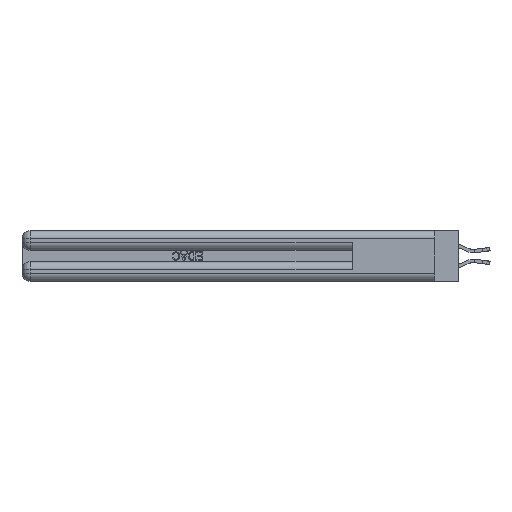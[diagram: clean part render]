
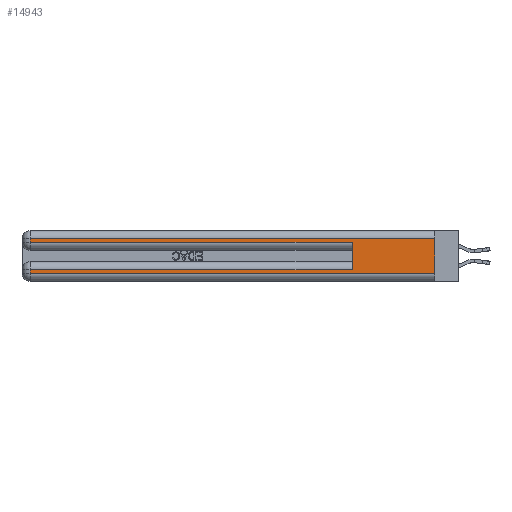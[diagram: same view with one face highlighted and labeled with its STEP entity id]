
A CAD part, left-side view. The second image highlights one B-rep face of the part: STEP entity #14943.
In plain terms, the highlighted planar face has unit normal (-1, 0, 0).
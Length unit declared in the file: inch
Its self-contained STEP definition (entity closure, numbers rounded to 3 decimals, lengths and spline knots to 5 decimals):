
#1509 = PLANE ( 'NONE',  #8215 ) ;
#1601 = CARTESIAN_POINT ( 'NONE',  ( 0., 0.6, 0.285 ) ) ;
#3131 = ORIENTED_EDGE ( 'NONE', *, *, #14412, .T. ) ;
#4865 = DIRECTION ( 'NONE',  ( 0., 0., -1. ) ) ;
#5297 = CARTESIAN_POINT ( 'NONE',  ( 0., 2.94, 0.285 ) ) ;
#6395 = CARTESIAN_POINT ( 'NONE',  ( 0., 2.94, 0.31 ) ) ;
#7022 = LINE ( 'NONE', #25173, #30333 ) ;
#7098 = CARTESIAN_POINT ( 'NONE',  ( 0., 0., 0.31 ) ) ;
#8215 = AXIS2_PLACEMENT_3D ( 'NONE', #33923, #28074, #10633 ) ;
#8663 = CARTESIAN_POINT ( 'NONE',  ( 0., 0., 0.06 ) ) ;
#8748 = VECTOR ( 'NONE', #35801, 39.37008 ) ;
#9563 = LINE ( 'NONE', #30442, #38534 ) ;
#9799 = FACE_OUTER_BOUND ( 'NONE', #31549, .T. ) ;
#10083 = DIRECTION ( 'NONE',  ( 0., 1., 0. ) ) ;
#10345 = ORIENTED_EDGE ( 'NONE', *, *, #35963, .T. ) ;
#10519 = DIRECTION ( 'NONE',  ( 0., 0., -1. ) ) ;
#10633 = DIRECTION ( 'NONE',  ( 0., 0., -1. ) ) ;
#10879 = VERTEX_POINT ( 'NONE', #28985 ) ;
#12045 = EDGE_CURVE ( 'NONE', #10879, #37387, #20792, .T. ) ;
#12166 = DIRECTION ( 'NONE',  ( 0., -1., 0. ) ) ;
#12324 = ORIENTED_EDGE ( 'NONE', *, *, #12874, .T. ) ;
#12874 = EDGE_CURVE ( 'NONE', #19707, #36325, #14661, .T. ) ;
#12913 = LINE ( 'NONE', #24014, #27831 ) ;
#13123 = ORIENTED_EDGE ( 'NONE', *, *, #16694, .T. ) ;
#13706 = EDGE_CURVE ( 'NONE', #19707, #15009, #23445, .T. ) ;
#13824 = CARTESIAN_POINT ( 'NONE',  ( 0., 0.6, 0.145 ) ) ;
#14403 = CARTESIAN_POINT ( 'NONE',  ( 0., 2.94, 0.085 ) ) ;
#14412 = EDGE_CURVE ( 'NONE', #36325, #10879, #7022, .T. ) ;
#14448 = CARTESIAN_POINT ( 'NONE',  ( 0., 0., 0.285 ) ) ;
#14661 = LINE ( 'NONE', #32530, #16981 ) ;
#14943 = ADVANCED_FACE ( 'NONE', ( #9799 ), #1509, .F. ) ;
#14963 = VERTEX_POINT ( 'NONE', #5297 ) ;
#15009 = VERTEX_POINT ( 'NONE', #1601 ) ;
#15499 = VECTOR ( 'NONE', #28806, 39.37008 ) ;
#16548 = DIRECTION ( 'NONE',  ( 0., 1., 0. ) ) ;
#16694 = EDGE_CURVE ( 'NONE', #14963, #15009, #17614, .T. ) ;
#16981 = VECTOR ( 'NONE', #16548, 39.37008 ) ;
#17614 = LINE ( 'NONE', #14448, #8748 ) ;
#18796 = VERTEX_POINT ( 'NONE', #6395 ) ;
#19657 = CARTESIAN_POINT ( 'NONE',  ( 0., 0.6, 0.085 ) ) ;
#19707 = VERTEX_POINT ( 'NONE', #19657 ) ;
#20143 = VERTEX_POINT ( 'NONE', #7098 ) ;
#20792 = LINE ( 'NONE', #8663, #28189 ) ;
#22022 = ORIENTED_EDGE ( 'NONE', *, *, #34890, .T. ) ;
#23445 = LINE ( 'NONE', #13824, #15499 ) ;
#24014 = CARTESIAN_POINT ( 'NONE',  ( 0., 2.94, 0.37 ) ) ;
#24496 = CARTESIAN_POINT ( 'NONE',  ( 0., 0., 0.37 ) ) ;
#25114 = ORIENTED_EDGE ( 'NONE', *, *, #13706, .F. ) ;
#25173 = CARTESIAN_POINT ( 'NONE',  ( 0., 2.94, 0.37 ) ) ;
#27245 = ORIENTED_EDGE ( 'NONE', *, *, #12045, .T. ) ;
#27779 = ORIENTED_EDGE ( 'NONE', *, *, #32619, .F. ) ;
#27831 = VECTOR ( 'NONE', #32738, 39.37008 ) ;
#28074 = DIRECTION ( 'NONE',  ( 1., 0., 0. ) ) ;
#28189 = VECTOR ( 'NONE', #12166, 39.37008 ) ;
#28806 = DIRECTION ( 'NONE',  ( 0., 0., 1. ) ) ;
#28985 = CARTESIAN_POINT ( 'NONE',  ( 0., 2.94, 0.06 ) ) ;
#30333 = VECTOR ( 'NONE', #4865, 39.37008 ) ;
#30442 = CARTESIAN_POINT ( 'NONE',  ( 0., 0., 0.31 ) ) ;
#31549 = EDGE_LOOP ( 'NONE', ( #27779, #10345, #22022, #13123, #25114, #12324, #3131, #27245 ) ) ;
#32530 = CARTESIAN_POINT ( 'NONE',  ( 0., 0., 0.085 ) ) ;
#32619 = EDGE_CURVE ( 'NONE', #20143, #37387, #32656, .T. ) ;
#32656 = LINE ( 'NONE', #24496, #36821 ) ;
#32738 = DIRECTION ( 'NONE',  ( 0., 0., -1. ) ) ;
#33923 = CARTESIAN_POINT ( 'NONE',  ( 0., 0., 0.37 ) ) ;
#34092 = CARTESIAN_POINT ( 'NONE',  ( 0., 0., 0.06 ) ) ;
#34890 = EDGE_CURVE ( 'NONE', #18796, #14963, #12913, .T. ) ;
#35801 = DIRECTION ( 'NONE',  ( 0., -1., 0. ) ) ;
#35963 = EDGE_CURVE ( 'NONE', #20143, #18796, #9563, .T. ) ;
#36325 = VERTEX_POINT ( 'NONE', #14403 ) ;
#36821 = VECTOR ( 'NONE', #10519, 39.37008 ) ;
#37387 = VERTEX_POINT ( 'NONE', #34092 ) ;
#38534 = VECTOR ( 'NONE', #10083, 39.37008 ) ;
